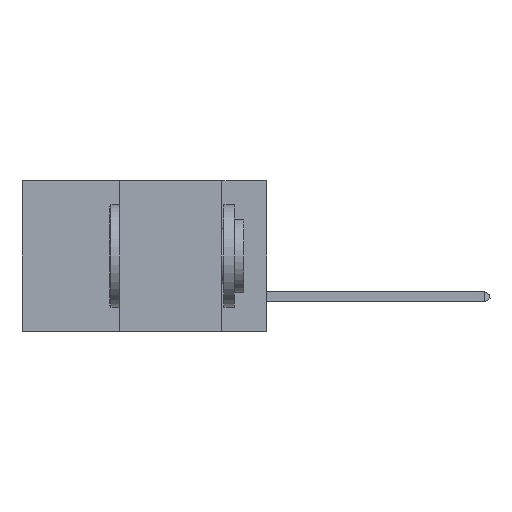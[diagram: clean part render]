
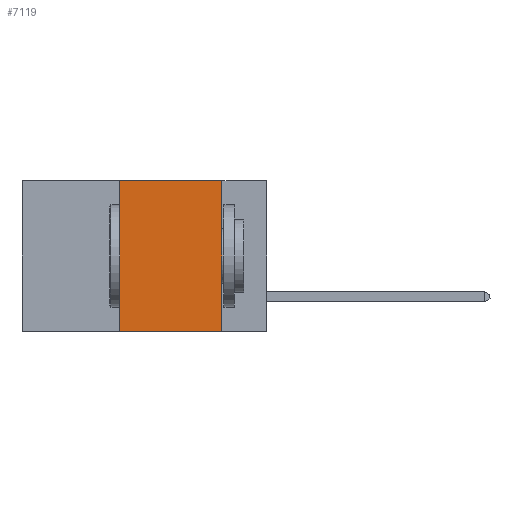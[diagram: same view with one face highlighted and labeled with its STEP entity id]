
A CAD part, left-side view. The second image highlights one B-rep face of the part: STEP entity #7119.
In plain terms, the highlighted planar face has unit normal (-1, 0, 0).
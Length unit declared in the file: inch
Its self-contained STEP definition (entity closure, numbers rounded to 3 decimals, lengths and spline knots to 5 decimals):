
#331 = VERTEX_POINT ( 'NONE', #7923 ) ;
#530 = CARTESIAN_POINT ( 'NONE',  ( 0., 0.11, 0. ) ) ;
#717 = ORIENTED_EDGE ( 'NONE', *, *, #8843, .F. ) ;
#749 = FACE_OUTER_BOUND ( 'NONE', #13452, .T. ) ;
#778 = DIRECTION ( 'NONE',  ( 0., 0., 1. ) ) ;
#859 = LINE ( 'NONE', #10888, #9086 ) ;
#1109 = DIRECTION ( 'NONE',  ( 0., -1., 0. ) ) ;
#1177 = CARTESIAN_POINT ( 'NONE',  ( 0., 0.11, 0. ) ) ;
#1851 = VECTOR ( 'NONE', #8761, 39.37008 ) ;
#2125 = ORIENTED_EDGE ( 'NONE', *, *, #10847, .T. ) ;
#2791 = ORIENTED_EDGE ( 'NONE', *, *, #10147, .F. ) ;
#3036 = CARTESIAN_POINT ( 'NONE',  ( 0., 0.36, 0. ) ) ;
#3169 = VERTEX_POINT ( 'NONE', #13079 ) ;
#4033 = ORIENTED_EDGE ( 'NONE', *, *, #4146, .F. ) ;
#4146 = EDGE_CURVE ( 'NONE', #4409, #331, #12618, .T. ) ;
#4147 = VERTEX_POINT ( 'NONE', #3036 ) ;
#4407 = DIRECTION ( 'NONE',  ( 0., 0., -1. ) ) ;
#4409 = VERTEX_POINT ( 'NONE', #1177 ) ;
#5968 = LINE ( 'NONE', #11718, #11750 ) ;
#6172 = VECTOR ( 'NONE', #778, 39.37008 ) ;
#7119 = ADVANCED_FACE ( 'NONE', ( #749 ), #8847, .F. ) ;
#7923 = CARTESIAN_POINT ( 'NONE',  ( 0., 0.11, -0.37 ) ) ;
#8761 = DIRECTION ( 'NONE',  ( 0., 0., -1. ) ) ;
#8843 = EDGE_CURVE ( 'NONE', #4147, #4409, #859, .T. ) ;
#8847 = PLANE ( 'NONE',  #9780 ) ;
#8861 = LINE ( 'NONE', #10069, #6172 ) ;
#9086 = VECTOR ( 'NONE', #11084, 39.37008 ) ;
#9780 = AXIS2_PLACEMENT_3D ( 'NONE', #12394, #14773, #4407 ) ;
#10069 = CARTESIAN_POINT ( 'NONE',  ( 0., 0.36, 0. ) ) ;
#10147 = EDGE_CURVE ( 'NONE', #3169, #4147, #8861, .T. ) ;
#10847 = EDGE_CURVE ( 'NONE', #3169, #331, #5968, .T. ) ;
#10888 = CARTESIAN_POINT ( 'NONE',  ( 0., 0.6, 0. ) ) ;
#11084 = DIRECTION ( 'NONE',  ( 0., -1., 0. ) ) ;
#11718 = CARTESIAN_POINT ( 'NONE',  ( 0., 0.6, -0.37 ) ) ;
#11750 = VECTOR ( 'NONE', #1109, 39.37008 ) ;
#12394 = CARTESIAN_POINT ( 'NONE',  ( 0., 0.6, 0. ) ) ;
#12618 = LINE ( 'NONE', #530, #1851 ) ;
#13079 = CARTESIAN_POINT ( 'NONE',  ( 0., 0.36, -0.37 ) ) ;
#13452 = EDGE_LOOP ( 'NONE', ( #4033, #717, #2791, #2125 ) ) ;
#14773 = DIRECTION ( 'NONE',  ( 1., 0., 0. ) ) ;
